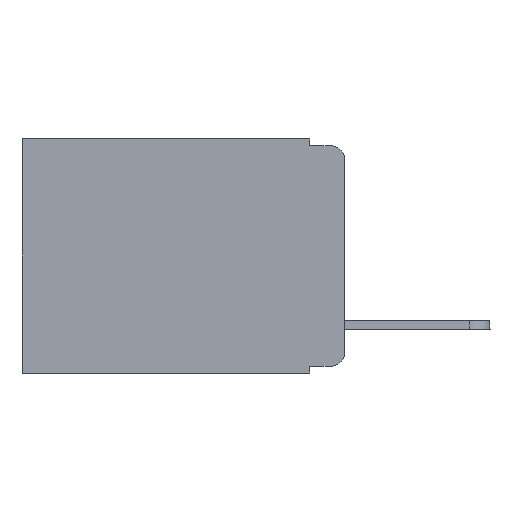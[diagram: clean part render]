
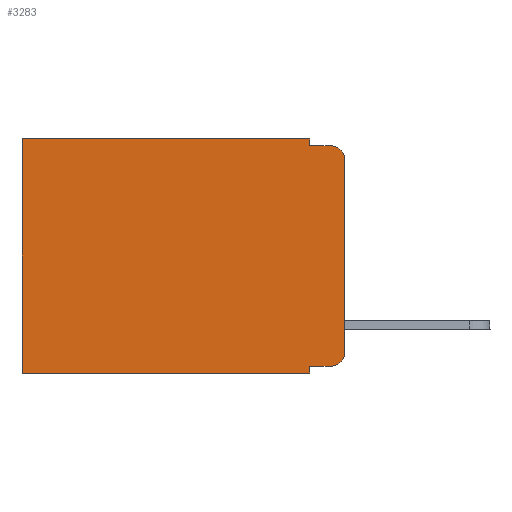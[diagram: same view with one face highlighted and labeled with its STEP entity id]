
A CAD part, left-side view. The second image highlights one B-rep face of the part: STEP entity #3283.
In plain terms, the highlighted planar face has unit normal (-1, 0, 0).
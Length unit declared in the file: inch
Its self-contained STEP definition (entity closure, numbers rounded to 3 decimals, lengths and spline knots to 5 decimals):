
#120 = VECTOR ( 'NONE', #15961, 39.37008 ) ;
#340 = DIRECTION ( 'NONE',  ( 0., 0., -1. ) ) ;
#689 = CARTESIAN_POINT ( 'NONE',  ( 0.298, 0.02, -0.313 ) ) ;
#1192 = DIRECTION ( 'NONE',  ( 0., -1., 0. ) ) ;
#1400 = VECTOR ( 'NONE', #12282, 39.37008 ) ;
#1478 = VECTOR ( 'NONE', #1192, 39.37008 ) ;
#2047 = ORIENTED_EDGE ( 'NONE', *, *, #15635, .F. ) ;
#2263 = CARTESIAN_POINT ( 'NONE',  ( 0.298, 0.051, -0.333 ) ) ;
#2308 = CARTESIAN_POINT ( 'NONE',  ( 0.298, 0., -0.343 ) ) ;
#2957 = ORIENTED_EDGE ( 'NONE', *, *, #11792, .T. ) ;
#3283 = ADVANCED_FACE ( 'NONE', ( #7046 ), #10823, .F. ) ;
#3668 = EDGE_CURVE ( 'NONE', #19208, #16474, #10553, .T. ) ;
#3697 = VECTOR ( 'NONE', #12805, 39.37008 ) ;
#3754 = EDGE_CURVE ( 'NONE', #4472, #16376, #7828, .T. ) ;
#3867 = CARTESIAN_POINT ( 'NONE',  ( 0.298, 0., 0. ) ) ;
#3945 = CARTESIAN_POINT ( 'NONE',  ( 0.298, 0.473, 0. ) ) ;
#4004 = ORIENTED_EDGE ( 'NONE', *, *, #3668, .F. ) ;
#4008 = VERTEX_POINT ( 'NONE', #7104 ) ;
#4472 = VERTEX_POINT ( 'NONE', #11178 ) ;
#4611 = DIRECTION ( 'NONE',  ( 0., -1., 0. ) ) ;
#4706 = VECTOR ( 'NONE', #4611, 39.37008 ) ;
#5255 = CARTESIAN_POINT ( 'NONE',  ( 0.298, 0.02, -0.01 ) ) ;
#5476 = CARTESIAN_POINT ( 'NONE',  ( 0.298, 0.02, -0.03 ) ) ;
#5589 = LINE ( 'NONE', #14790, #3697 ) ;
#6159 = DIRECTION ( 'NONE',  ( 0., 0., -1. ) ) ;
#6890 = VERTEX_POINT ( 'NONE', #7578 ) ;
#6899 = DIRECTION ( 'NONE',  ( 0., 0., -1. ) ) ;
#7046 = FACE_OUTER_BOUND ( 'NONE', #11351, .T. ) ;
#7104 = CARTESIAN_POINT ( 'NONE',  ( 0.298, 0.473, -0.343 ) ) ;
#7578 = CARTESIAN_POINT ( 'NONE',  ( 0.298, 0., -0.313 ) ) ;
#7579 = VERTEX_POINT ( 'NONE', #5255 ) ;
#7805 = CIRCLE ( 'NONE', #20993, 0.02 ) ;
#7828 = LINE ( 'NONE', #20122, #17488 ) ;
#7883 = CARTESIAN_POINT ( 'NONE',  ( 0.298, 0.02, -0.333 ) ) ;
#8477 = CARTESIAN_POINT ( 'NONE',  ( 0.298, 0., -0.03 ) ) ;
#9121 = CARTESIAN_POINT ( 'NONE',  ( 0.298, 0.051, -0.01 ) ) ;
#9160 = DIRECTION ( 'NONE',  ( 0., 0., -1. ) ) ;
#9635 = CARTESIAN_POINT ( 'NONE',  ( 0.298, 0., 0. ) ) ;
#10010 = CARTESIAN_POINT ( 'NONE',  ( 0.298, 0.051, -0.333 ) ) ;
#10062 = VERTEX_POINT ( 'NONE', #8477 ) ;
#10163 = ORIENTED_EDGE ( 'NONE', *, *, #20449, .F. ) ;
#10553 = LINE ( 'NONE', #21298, #15953 ) ;
#10823 = PLANE ( 'NONE',  #20114 ) ;
#11178 = CARTESIAN_POINT ( 'NONE',  ( 0.298, 0.051, 0. ) ) ;
#11351 = EDGE_LOOP ( 'NONE', ( #2047, #16012, #10163, #13833, #2957, #11452, #21977, #4004, #11678, #15192 ) ) ;
#11452 = ORIENTED_EDGE ( 'NONE', *, *, #19897, .T. ) ;
#11678 = ORIENTED_EDGE ( 'NONE', *, *, #15076, .T. ) ;
#11792 = EDGE_CURVE ( 'NONE', #4472, #17645, #17991, .T. ) ;
#12282 = DIRECTION ( 'NONE',  ( 0., 1., 0. ) ) ;
#12679 = DIRECTION ( 'NONE',  ( 0., 0., -1. ) ) ;
#12805 = DIRECTION ( 'NONE',  ( 0., 0., -1. ) ) ;
#13525 = LINE ( 'NONE', #9635, #15236 ) ;
#13833 = ORIENTED_EDGE ( 'NONE', *, *, #3754, .F. ) ;
#13914 = VERTEX_POINT ( 'NONE', #7883 ) ;
#14790 = CARTESIAN_POINT ( 'NONE',  ( 0.298, 0.473, 0. ) ) ;
#15006 = CARTESIAN_POINT ( 'NONE',  ( 0.298, 0.051, -0.343 ) ) ;
#15076 = EDGE_CURVE ( 'NONE', #19208, #13914, #17112, .T. ) ;
#15192 = ORIENTED_EDGE ( 'NONE', *, *, #19452, .T. ) ;
#15236 = VECTOR ( 'NONE', #20731, 39.37008 ) ;
#15309 = CARTESIAN_POINT ( 'NONE',  ( 0.298, 0.051, -0.01 ) ) ;
#15635 = EDGE_CURVE ( 'NONE', #10062, #6890, #13525, .T. ) ;
#15694 = CIRCLE ( 'NONE', #18337, 0.02 ) ;
#15953 = VECTOR ( 'NONE', #6899, 39.37008 ) ;
#15961 = DIRECTION ( 'NONE',  ( 0., 1., 0. ) ) ;
#16012 = ORIENTED_EDGE ( 'NONE', *, *, #18937, .T. ) ;
#16090 = CARTESIAN_POINT ( 'NONE',  ( 0.298, 0., 0. ) ) ;
#16376 = VERTEX_POINT ( 'NONE', #9121 ) ;
#16474 = VERTEX_POINT ( 'NONE', #15006 ) ;
#17112 = LINE ( 'NONE', #10010, #4706 ) ;
#17488 = VECTOR ( 'NONE', #6159, 39.37008 ) ;
#17645 = VERTEX_POINT ( 'NONE', #3945 ) ;
#17991 = LINE ( 'NONE', #16090, #120 ) ;
#18221 = DIRECTION ( 'NONE',  ( -1., 0., 0. ) ) ;
#18257 = DIRECTION ( 'NONE',  ( -1., 0., 0. ) ) ;
#18337 = AXIS2_PLACEMENT_3D ( 'NONE', #5476, #18221, #12679 ) ;
#18937 = EDGE_CURVE ( 'NONE', #10062, #7579, #15694, .T. ) ;
#18952 = EDGE_CURVE ( 'NONE', #16474, #4008, #21987, .T. ) ;
#19208 = VERTEX_POINT ( 'NONE', #2263 ) ;
#19333 = LINE ( 'NONE', #15309, #1478 ) ;
#19452 = EDGE_CURVE ( 'NONE', #13914, #6890, #7805, .T. ) ;
#19673 = DIRECTION ( 'NONE',  ( 1., 0., 0. ) ) ;
#19897 = EDGE_CURVE ( 'NONE', #17645, #4008, #5589, .T. ) ;
#20114 = AXIS2_PLACEMENT_3D ( 'NONE', #3867, #19673, #9160 ) ;
#20122 = CARTESIAN_POINT ( 'NONE',  ( 0.298, 0.051, 0. ) ) ;
#20449 = EDGE_CURVE ( 'NONE', #16376, #7579, #19333, .T. ) ;
#20731 = DIRECTION ( 'NONE',  ( 0., 0., -1. ) ) ;
#20993 = AXIS2_PLACEMENT_3D ( 'NONE', #689, #18257, #340 ) ;
#21298 = CARTESIAN_POINT ( 'NONE',  ( 0.298, 0.051, 0. ) ) ;
#21977 = ORIENTED_EDGE ( 'NONE', *, *, #18952, .F. ) ;
#21987 = LINE ( 'NONE', #2308, #1400 ) ;
